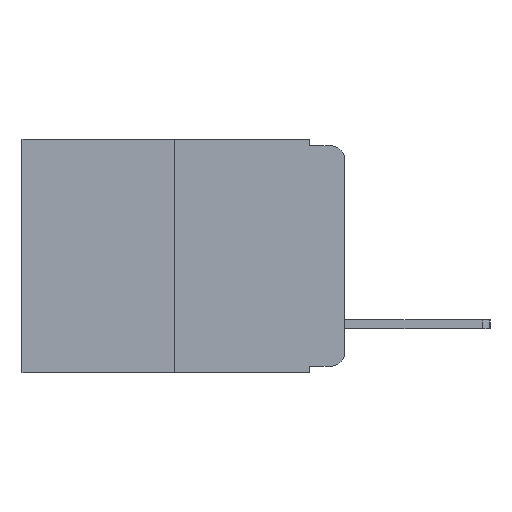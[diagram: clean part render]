
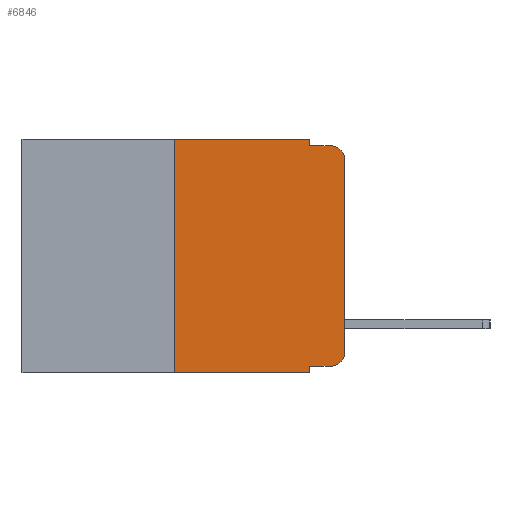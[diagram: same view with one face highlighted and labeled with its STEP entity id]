
A CAD part, left-side view. The second image highlights one B-rep face of the part: STEP entity #6846.
In plain terms, the highlighted planar face has unit normal (-1, 0, 0).
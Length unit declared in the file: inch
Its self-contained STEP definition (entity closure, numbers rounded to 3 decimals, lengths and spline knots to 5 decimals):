
#103 = CARTESIAN_POINT ( 'NONE',  ( 0., 0.473, 0. ) ) ;
#755 = EDGE_CURVE ( 'NONE', #2249, #6722, #4615, .T. ) ;
#1804 = VECTOR ( 'NONE', #8985, 39.37008 ) ;
#2022 = CARTESIAN_POINT ( 'NONE',  ( 0., 0.051, -0.01 ) ) ;
#2052 = ORIENTED_EDGE ( 'NONE', *, *, #10672, .F. ) ;
#2059 = CARTESIAN_POINT ( 'NONE',  ( 0., 0.051, 0. ) ) ;
#2148 = DIRECTION ( 'NONE',  ( 0., 0., -1. ) ) ;
#2149 = EDGE_CURVE ( 'NONE', #6896, #11509, #6826, .T. ) ;
#2249 = VERTEX_POINT ( 'NONE', #11065 ) ;
#2801 = EDGE_CURVE ( 'NONE', #8236, #13483, #13653, .T. ) ;
#3592 = LINE ( 'NONE', #2022, #13736 ) ;
#3857 = LINE ( 'NONE', #10814, #13593 ) ;
#3861 = DIRECTION ( 'NONE',  ( -1., 0., 0. ) ) ;
#4057 = DIRECTION ( 'NONE',  ( 1., 0., 0. ) ) ;
#4170 = CARTESIAN_POINT ( 'NONE',  ( 0., 0.25, -0.343 ) ) ;
#4297 = ORIENTED_EDGE ( 'NONE', *, *, #4366, .T. ) ;
#4334 = VERTEX_POINT ( 'NONE', #9189 ) ;
#4366 = EDGE_CURVE ( 'NONE', #13483, #4334, #3857, .T. ) ;
#4520 = LINE ( 'NONE', #15981, #11016 ) ;
#4571 = EDGE_CURVE ( 'NONE', #9733, #8236, #8332, .T. ) ;
#4615 = LINE ( 'NONE', #2059, #14300 ) ;
#4718 = ORIENTED_EDGE ( 'NONE', *, *, #6001, .F. ) ;
#5131 = ORIENTED_EDGE ( 'NONE', *, *, #9608, .F. ) ;
#5135 = CARTESIAN_POINT ( 'NONE',  ( 0., 0., -0.313 ) ) ;
#5382 = CARTESIAN_POINT ( 'NONE',  ( 0., 0.25, 0. ) ) ;
#5542 = ORIENTED_EDGE ( 'NONE', *, *, #2149, .T. ) ;
#5581 = VECTOR ( 'NONE', #5956, 39.37008 ) ;
#5824 = CARTESIAN_POINT ( 'NONE',  ( 0., 0.473, -0.343 ) ) ;
#5956 = DIRECTION ( 'NONE',  ( 0., -1., 0. ) ) ;
#6001 = EDGE_CURVE ( 'NONE', #6722, #6121, #3592, .T. ) ;
#6121 = VERTEX_POINT ( 'NONE', #6266 ) ;
#6266 = CARTESIAN_POINT ( 'NONE',  ( 0., 0.02, -0.01 ) ) ;
#6722 = VERTEX_POINT ( 'NONE', #12723 ) ;
#6826 = LINE ( 'NONE', #5824, #5581 ) ;
#6846 = ADVANCED_FACE ( 'NONE', ( #14844 ), #7934, .F. ) ;
#6896 = VERTEX_POINT ( 'NONE', #4170 ) ;
#7000 = CIRCLE ( 'NONE', #14169, 0.02 ) ;
#7157 = DIRECTION ( 'NONE',  ( 0., 0., -1. ) ) ;
#7194 = EDGE_CURVE ( 'NONE', #9733, #11509, #13136, .T. ) ;
#7934 = PLANE ( 'NONE',  #8344 ) ;
#8236 = VERTEX_POINT ( 'NONE', #9493 ) ;
#8254 = DIRECTION ( 'NONE',  ( 0., 0., 1. ) ) ;
#8332 = LINE ( 'NONE', #11036, #1804 ) ;
#8344 = AXIS2_PLACEMENT_3D ( 'NONE', #103, #4057, #12990 ) ;
#8557 = LINE ( 'NONE', #15636, #11895 ) ;
#8671 = CARTESIAN_POINT ( 'NONE',  ( 0., 0.051, 0. ) ) ;
#8846 = DIRECTION ( 'NONE',  ( -1., 0., 0. ) ) ;
#8865 = CARTESIAN_POINT ( 'NONE',  ( 0., 0.02, -0.313 ) ) ;
#8930 = CARTESIAN_POINT ( 'NONE',  ( 0., 0.051, -0.343 ) ) ;
#8985 = DIRECTION ( 'NONE',  ( 0., -1., 0. ) ) ;
#9014 = ORIENTED_EDGE ( 'NONE', *, *, #7194, .F. ) ;
#9189 = CARTESIAN_POINT ( 'NONE',  ( 0., 0., -0.03 ) ) ;
#9404 = ORIENTED_EDGE ( 'NONE', *, *, #2801, .T. ) ;
#9405 = DIRECTION ( 'NONE',  ( 0., 0., 1. ) ) ;
#9493 = CARTESIAN_POINT ( 'NONE',  ( 0., 0.02, -0.333 ) ) ;
#9608 = EDGE_CURVE ( 'NONE', #15232, #2249, #4520, .T. ) ;
#9733 = VERTEX_POINT ( 'NONE', #12734 ) ;
#9845 = DIRECTION ( 'NONE',  ( 0., -1., 0. ) ) ;
#9887 = VECTOR ( 'NONE', #2148, 39.37008 ) ;
#10672 = EDGE_CURVE ( 'NONE', #6896, #15232, #8557, .T. ) ;
#10814 = CARTESIAN_POINT ( 'NONE',  ( 0., 0., 0. ) ) ;
#11016 = VECTOR ( 'NONE', #11323, 39.37008 ) ;
#11036 = CARTESIAN_POINT ( 'NONE',  ( 0., 0.051, -0.333 ) ) ;
#11065 = CARTESIAN_POINT ( 'NONE',  ( 0., 0.051, 0. ) ) ;
#11323 = DIRECTION ( 'NONE',  ( 0., -1., 0. ) ) ;
#11509 = VERTEX_POINT ( 'NONE', #8930 ) ;
#11581 = CARTESIAN_POINT ( 'NONE',  ( 0., 0.02, -0.03 ) ) ;
#11895 = VECTOR ( 'NONE', #8254, 39.37008 ) ;
#12723 = CARTESIAN_POINT ( 'NONE',  ( 0., 0.051, -0.01 ) ) ;
#12734 = CARTESIAN_POINT ( 'NONE',  ( 0., 0.051, -0.333 ) ) ;
#12797 = DIRECTION ( 'NONE',  ( 0., 0., -1. ) ) ;
#12990 = DIRECTION ( 'NONE',  ( 0., 0., -1. ) ) ;
#13136 = LINE ( 'NONE', #8671, #9887 ) ;
#13483 = VERTEX_POINT ( 'NONE', #5135 ) ;
#13523 = AXIS2_PLACEMENT_3D ( 'NONE', #8865, #8846, #7157 ) ;
#13593 = VECTOR ( 'NONE', #9405, 39.37008 ) ;
#13653 = CIRCLE ( 'NONE', #13523, 0.02 ) ;
#13736 = VECTOR ( 'NONE', #9845, 39.37008 ) ;
#14169 = AXIS2_PLACEMENT_3D ( 'NONE', #11581, #3861, #12797 ) ;
#14300 = VECTOR ( 'NONE', #16021, 39.37008 ) ;
#14402 = ORIENTED_EDGE ( 'NONE', *, *, #14525, .T. ) ;
#14525 = EDGE_CURVE ( 'NONE', #4334, #6121, #7000, .T. ) ;
#14767 = ORIENTED_EDGE ( 'NONE', *, *, #755, .F. ) ;
#14823 = EDGE_LOOP ( 'NONE', ( #4297, #14402, #4718, #14767, #5131, #2052, #5542, #9014, #15515, #9404 ) ) ;
#14844 = FACE_OUTER_BOUND ( 'NONE', #14823, .T. ) ;
#15232 = VERTEX_POINT ( 'NONE', #5382 ) ;
#15515 = ORIENTED_EDGE ( 'NONE', *, *, #4571, .T. ) ;
#15636 = CARTESIAN_POINT ( 'NONE',  ( 0., 0.25, 0. ) ) ;
#15981 = CARTESIAN_POINT ( 'NONE',  ( 0., 0.473, 0. ) ) ;
#16021 = DIRECTION ( 'NONE',  ( 0., 0., -1. ) ) ;
